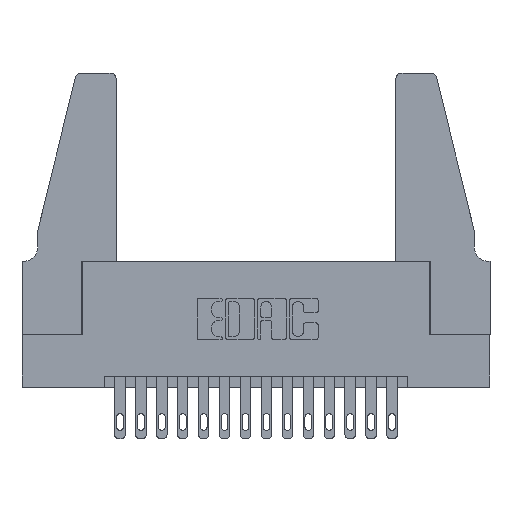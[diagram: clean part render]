
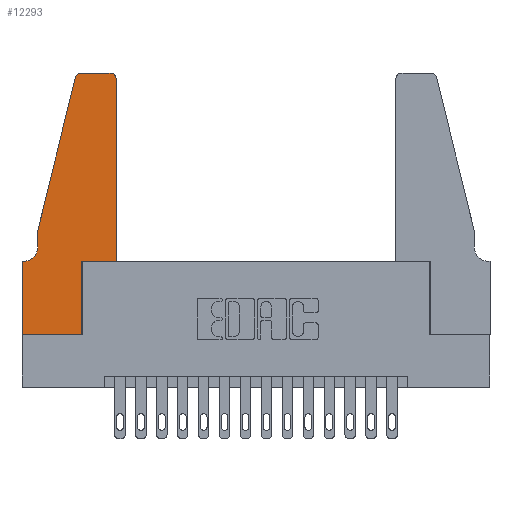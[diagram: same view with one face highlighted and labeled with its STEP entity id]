
A CAD part, top view. The second image highlights one B-rep face of the part: STEP entity #12293.
In plain terms, the highlighted planar face has unit normal (0, 0, 1).
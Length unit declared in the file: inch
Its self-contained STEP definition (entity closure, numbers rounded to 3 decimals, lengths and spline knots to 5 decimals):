
#226 = ORIENTED_EDGE ( 'NONE', *, *, #7484, .T. ) ;
#388 = LINE ( 'NONE', #15707, #12194 ) ;
#397 = CARTESIAN_POINT ( 'NONE',  ( 0.284, 1.25, 0.37 ) ) ;
#437 = ORIENTED_EDGE ( 'NONE', *, *, #11648, .T. ) ;
#478 = CARTESIAN_POINT ( 'NONE',  ( 0.0755, 0.42, 0.37 ) ) ;
#541 = ORIENTED_EDGE ( 'NONE', *, *, #16036, .T. ) ;
#928 = ORIENTED_EDGE ( 'NONE', *, *, #9996, .T. ) ;
#1262 = LINE ( 'NONE', #15227, #14507 ) ;
#1385 = CARTESIAN_POINT ( 'NONE',  ( 0.0755, 0.5, 0.37 ) ) ;
#1392 = LINE ( 'NONE', #10390, #12780 ) ;
#1452 = DIRECTION ( 'NONE',  ( -0.239, -0.971, 0. ) ) ;
#1508 = CARTESIAN_POINT ( 'NONE',  ( 0.25487, 1.22718, 0.37 ) ) ;
#1639 = DIRECTION ( 'NONE',  ( 0., -1., 0. ) ) ;
#1871 = VECTOR ( 'NONE', #13926, 39.37008 ) ;
#2075 = LINE ( 'NONE', #13871, #1871 ) ;
#2188 = VERTEX_POINT ( 'NONE', #11434 ) ;
#2583 = ORIENTED_EDGE ( 'NONE', *, *, #12756, .T. ) ;
#2870 = ORIENTED_EDGE ( 'NONE', *, *, #5286, .T. ) ;
#2972 = CARTESIAN_POINT ( 'NONE',  ( 0., 0., 0.37 ) ) ;
#3037 = ORIENTED_EDGE ( 'NONE', *, *, #11938, .T. ) ;
#3284 = CIRCLE ( 'NONE', #11312, 0.03 ) ;
#3908 = DIRECTION ( 'NONE',  ( 0., 0., 1. ) ) ;
#3946 = VERTEX_POINT ( 'NONE', #16234 ) ;
#4220 = PLANE ( 'NONE',  #15963 ) ;
#4537 = VERTEX_POINT ( 'NONE', #15326 ) ;
#4569 = DIRECTION ( 'NONE',  ( -1., 0., 0. ) ) ;
#4776 = CARTESIAN_POINT ( 'NONE',  ( 0., 0.35, 0.37 ) ) ;
#4865 = LINE ( 'NONE', #15309, #8356 ) ;
#5083 = CIRCLE ( 'NONE', #8424, 0.03 ) ;
#5286 = EDGE_CURVE ( 'NONE', #3946, #7376, #388, .T. ) ;
#5407 = LINE ( 'NONE', #10572, #7449 ) ;
#6344 = ORIENTED_EDGE ( 'NONE', *, *, #12659, .T. ) ;
#6665 = CARTESIAN_POINT ( 'NONE',  ( 0.4205, 1.22, 0.37 ) ) ;
#6687 = EDGE_LOOP ( 'NONE', ( #226, #6344, #7858, #541, #11697, #437, #928, #2583, #3037, #12925, #2870, #10543 ) ) ;
#6713 = EDGE_CURVE ( 'NONE', #7376, #2188, #3284, .T. ) ;
#7071 = CARTESIAN_POINT ( 'NONE',  ( 0.2865, 0.35, 0.37 ) ) ;
#7077 = CARTESIAN_POINT ( 'NONE',  ( 0.0755, 0.35, 0.37 ) ) ;
#7331 = VERTEX_POINT ( 'NONE', #397 ) ;
#7376 = VERTEX_POINT ( 'NONE', #12124 ) ;
#7449 = VECTOR ( 'NONE', #1639, 39.37008 ) ;
#7479 = EDGE_CURVE ( 'NONE', #15301, #8611, #16110, .T. ) ;
#7484 = EDGE_CURVE ( 'NONE', #2188, #7331, #15106, .T. ) ;
#7639 = CARTESIAN_POINT ( 'NONE',  ( 0.0055, 0.35, 0.37 ) ) ;
#7858 = ORIENTED_EDGE ( 'NONE', *, *, #13720, .T. ) ;
#8054 = DIRECTION ( 'NONE',  ( 1., 0., 0. ) ) ;
#8099 = DIRECTION ( 'NONE',  ( 0., 0., 1. ) ) ;
#8133 = DIRECTION ( 'NONE',  ( 1., 0., 0. ) ) ;
#8356 = VECTOR ( 'NONE', #16596, 39.37008 ) ;
#8424 = AXIS2_PLACEMENT_3D ( 'NONE', #12562, #11033, #9803 ) ;
#8474 = CARTESIAN_POINT ( 'NONE',  ( 0.2605, 1.25, 0.37 ) ) ;
#8527 = VERTEX_POINT ( 'NONE', #9523 ) ;
#8611 = VERTEX_POINT ( 'NONE', #7639 ) ;
#8839 = EDGE_CURVE ( 'NONE', #16570, #3946, #4865, .T. ) ;
#9080 = VECTOR ( 'NONE', #13768, 39.37008 ) ;
#9353 = DIRECTION ( 'NONE',  ( 0., 1., 0. ) ) ;
#9523 = CARTESIAN_POINT ( 'NONE',  ( 0., 0.35, 0.37 ) ) ;
#9698 = LINE ( 'NONE', #7077, #9080 ) ;
#9803 = DIRECTION ( 'NONE',  ( 1., 0., 0. ) ) ;
#9866 = DIRECTION ( 'NONE',  ( 0., 0., -1. ) ) ;
#9996 = EDGE_CURVE ( 'NONE', #8527, #11842, #1392, .T. ) ;
#9997 = DIRECTION ( 'NONE',  ( 1., 0., 0. ) ) ;
#10390 = CARTESIAN_POINT ( 'NONE',  ( 0., 0., 0.37 ) ) ;
#10543 = ORIENTED_EDGE ( 'NONE', *, *, #6713, .T. ) ;
#10572 = CARTESIAN_POINT ( 'NONE',  ( 0.0755, 0.5, 0.37 ) ) ;
#10869 = VERTEX_POINT ( 'NONE', #1508 ) ;
#11033 = DIRECTION ( 'NONE',  ( 0., 0., 1. ) ) ;
#11254 = FACE_OUTER_BOUND ( 'NONE', #6687, .T. ) ;
#11312 = AXIS2_PLACEMENT_3D ( 'NONE', #6665, #8099, #8054 ) ;
#11434 = CARTESIAN_POINT ( 'NONE',  ( 0.4205, 1.25, 0.37 ) ) ;
#11435 = LINE ( 'NONE', #1385, #16726 ) ;
#11648 = EDGE_CURVE ( 'NONE', #8611, #8527, #9698, .T. ) ;
#11697 = ORIENTED_EDGE ( 'NONE', *, *, #7479, .T. ) ;
#11842 = VERTEX_POINT ( 'NONE', #2972 ) ;
#11938 = EDGE_CURVE ( 'NONE', #4537, #16570, #2075, .T. ) ;
#12124 = CARTESIAN_POINT ( 'NONE',  ( 0.4505, 1.22, 0.37 ) ) ;
#12194 = VECTOR ( 'NONE', #9353, 39.37008 ) ;
#12293 = ADVANCED_FACE ( 'NONE', ( #11254 ), #4220, .T. ) ;
#12456 = DIRECTION ( 'NONE',  ( -1., 0., 0. ) ) ;
#12562 = CARTESIAN_POINT ( 'NONE',  ( 0.284, 1.22, 0.37 ) ) ;
#12659 = EDGE_CURVE ( 'NONE', #7331, #10869, #5083, .T. ) ;
#12756 = EDGE_CURVE ( 'NONE', #11842, #4537, #1262, .T. ) ;
#12780 = VECTOR ( 'NONE', #14263, 39.37008 ) ;
#12925 = ORIENTED_EDGE ( 'NONE', *, *, #8839, .T. ) ;
#13459 = CARTESIAN_POINT ( 'NONE',  ( 0.0755, 0.5, 0.37 ) ) ;
#13481 = VERTEX_POINT ( 'NONE', #13459 ) ;
#13720 = EDGE_CURVE ( 'NONE', #10869, #13481, #11435, .T. ) ;
#13763 = CARTESIAN_POINT ( 'NONE',  ( 0.0055, 0.42, 0.37 ) ) ;
#13768 = DIRECTION ( 'NONE',  ( -1., 0., 0. ) ) ;
#13871 = CARTESIAN_POINT ( 'NONE',  ( 0.2865, 0.35, 0.37 ) ) ;
#13891 = VECTOR ( 'NONE', #12456, 39.37008 ) ;
#13926 = DIRECTION ( 'NONE',  ( 0., 1., 0. ) ) ;
#14263 = DIRECTION ( 'NONE',  ( 0., -1., 0. ) ) ;
#14507 = VECTOR ( 'NONE', #9997, 39.37008 ) ;
#15106 = LINE ( 'NONE', #8474, #13891 ) ;
#15227 = CARTESIAN_POINT ( 'NONE',  ( 0., 0., 0.37 ) ) ;
#15301 = VERTEX_POINT ( 'NONE', #478 ) ;
#15309 = CARTESIAN_POINT ( 'NONE',  ( 0.4505, 0.35, 0.37 ) ) ;
#15326 = CARTESIAN_POINT ( 'NONE',  ( 0.2865, 0., 0.37 ) ) ;
#15578 = AXIS2_PLACEMENT_3D ( 'NONE', #13763, #9866, #4569 ) ;
#15707 = CARTESIAN_POINT ( 'NONE',  ( 0.4505, 0.35, 0.37 ) ) ;
#15963 = AXIS2_PLACEMENT_3D ( 'NONE', #4776, #3908, #8133 ) ;
#16036 = EDGE_CURVE ( 'NONE', #13481, #15301, #5407, .T. ) ;
#16110 = CIRCLE ( 'NONE', #15578, 0.07 ) ;
#16234 = CARTESIAN_POINT ( 'NONE',  ( 0.4505, 0.35, 0.37 ) ) ;
#16570 = VERTEX_POINT ( 'NONE', #7071 ) ;
#16596 = DIRECTION ( 'NONE',  ( 1., 0., 0. ) ) ;
#16726 = VECTOR ( 'NONE', #1452, 39.37008 ) ;
